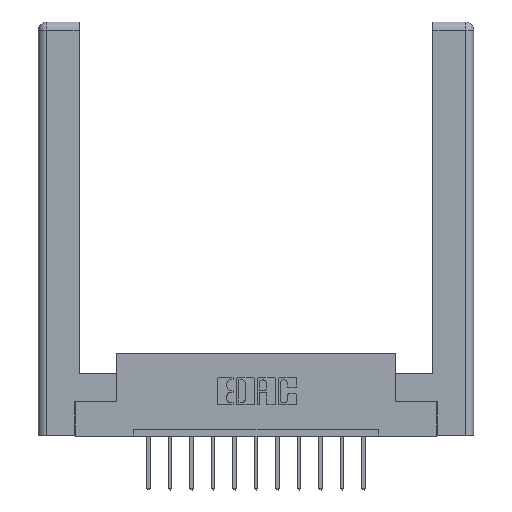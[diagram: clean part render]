
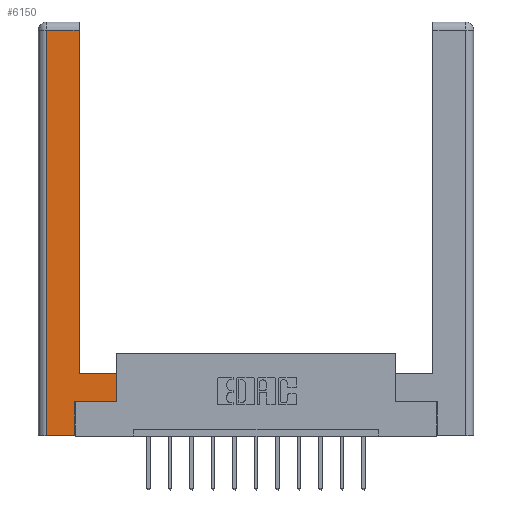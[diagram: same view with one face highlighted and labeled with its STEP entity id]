
A CAD part, top view. The second image highlights one B-rep face of the part: STEP entity #6150.
In plain terms, the highlighted planar face has unit normal (0, 0, 1).
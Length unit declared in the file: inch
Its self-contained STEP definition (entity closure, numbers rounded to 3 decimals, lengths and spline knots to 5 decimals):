
#1 = CARTESIAN_POINT ( 'NONE',  ( 0.295, 0.45, 0. ) ) ;
#195 = VERTEX_POINT ( 'NONE', #8451 ) ;
#566 = EDGE_CURVE ( 'NONE', #4747, #195, #12409, .T. ) ;
#671 = CARTESIAN_POINT ( 'NONE',  ( 0.565, 0.245, 0. ) ) ;
#918 = DIRECTION ( 'NONE',  ( -1., 0., 0. ) ) ;
#1179 = CARTESIAN_POINT ( 'NONE',  ( 0.265, 0.245, 0. ) ) ;
#1441 = EDGE_CURVE ( 'NONE', #195, #9207, #11475, .T. ) ;
#1463 = CARTESIAN_POINT ( 'NONE',  ( 0.0615, 0., 0. ) ) ;
#1494 = FACE_OUTER_BOUND ( 'NONE', #4042, .T. ) ;
#1576 = DIRECTION ( 'NONE',  ( 0., 1., 0. ) ) ;
#1592 = EDGE_CURVE ( 'NONE', #11965, #6570, #11661, .T. ) ;
#2027 = AXIS2_PLACEMENT_3D ( 'NONE', #5124, #5172, #2768 ) ;
#2190 = VECTOR ( 'NONE', #13616, 39.37008 ) ;
#2274 = EDGE_CURVE ( 'NONE', #11359, #4632, #4738, .T. ) ;
#2334 = VECTOR ( 'NONE', #12457, 39.37008 ) ;
#2402 = ORIENTED_EDGE ( 'NONE', *, *, #6427, .T. ) ;
#2768 = DIRECTION ( 'NONE',  ( -1., 0., 0. ) ) ;
#3490 = EDGE_CURVE ( 'NONE', #9207, #11965, #5975, .T. ) ;
#3733 = CARTESIAN_POINT ( 'NONE',  ( 0.295, 2.94, 0. ) ) ;
#4014 = ORIENTED_EDGE ( 'NONE', *, *, #566, .T. ) ;
#4042 = EDGE_LOOP ( 'NONE', ( #11072, #14363, #2402, #10550, #4014, #4528, #12501, #4617 ) ) ;
#4528 = ORIENTED_EDGE ( 'NONE', *, *, #1441, .T. ) ;
#4617 = ORIENTED_EDGE ( 'NONE', *, *, #1592, .T. ) ;
#4632 = VERTEX_POINT ( 'NONE', #6209 ) ;
#4738 = LINE ( 'NONE', #14704, #9374 ) ;
#4747 = VERTEX_POINT ( 'NONE', #6353 ) ;
#4816 = CARTESIAN_POINT ( 'NONE',  ( 0.295, 3., 0. ) ) ;
#4964 = LINE ( 'NONE', #6966, #10323 ) ;
#5046 = LINE ( 'NONE', #12704, #6117 ) ;
#5124 = CARTESIAN_POINT ( 'NONE',  ( 0., 0., 0. ) ) ;
#5172 = DIRECTION ( 'NONE',  ( 0., 0., -1. ) ) ;
#5835 = DIRECTION ( 'NONE',  ( 0., -1., 0. ) ) ;
#5836 = CARTESIAN_POINT ( 'NONE',  ( 0.565, 0.245, 0. ) ) ;
#5927 = PLANE ( 'NONE',  #2027 ) ;
#5975 = LINE ( 'NONE', #11966, #9903 ) ;
#6007 = CARTESIAN_POINT ( 'NONE',  ( 0.565, 0.45, 0. ) ) ;
#6117 = VECTOR ( 'NONE', #5835, 39.37008 ) ;
#6150 = ADVANCED_FACE ( 'NONE', ( #1494 ), #5927, .F. ) ;
#6209 = CARTESIAN_POINT ( 'NONE',  ( 0.0615, 2.94, 0. ) ) ;
#6353 = CARTESIAN_POINT ( 'NONE',  ( 0.265, 0., 0. ) ) ;
#6427 = EDGE_CURVE ( 'NONE', #4632, #9365, #5046, .T. ) ;
#6442 = VECTOR ( 'NONE', #7514, 39.37008 ) ;
#6570 = VERTEX_POINT ( 'NONE', #9885 ) ;
#6966 = CARTESIAN_POINT ( 'NONE',  ( 0.265, 0., 0. ) ) ;
#7514 = DIRECTION ( 'NONE',  ( 1., 0., 0. ) ) ;
#8451 = CARTESIAN_POINT ( 'NONE',  ( 0.265, 0.245, 0. ) ) ;
#9188 = VECTOR ( 'NONE', #9263, 39.37008 ) ;
#9207 = VERTEX_POINT ( 'NONE', #5836 ) ;
#9209 = EDGE_CURVE ( 'NONE', #6570, #11359, #12267, .T. ) ;
#9263 = DIRECTION ( 'NONE',  ( 0., 1., 0. ) ) ;
#9365 = VERTEX_POINT ( 'NONE', #1463 ) ;
#9374 = VECTOR ( 'NONE', #918, 39.37008 ) ;
#9885 = CARTESIAN_POINT ( 'NONE',  ( 0.295, 0.45, 0. ) ) ;
#9903 = VECTOR ( 'NONE', #1576, 39.37008 ) ;
#10323 = VECTOR ( 'NONE', #12722, 39.37008 ) ;
#10550 = ORIENTED_EDGE ( 'NONE', *, *, #14057, .T. ) ;
#11072 = ORIENTED_EDGE ( 'NONE', *, *, #9209, .T. ) ;
#11359 = VERTEX_POINT ( 'NONE', #3733 ) ;
#11475 = LINE ( 'NONE', #671, #6442 ) ;
#11661 = LINE ( 'NONE', #1, #2334 ) ;
#11965 = VERTEX_POINT ( 'NONE', #6007 ) ;
#11966 = CARTESIAN_POINT ( 'NONE',  ( 0.565, 0.45, 0. ) ) ;
#12267 = LINE ( 'NONE', #4816, #9188 ) ;
#12409 = LINE ( 'NONE', #1179, #2190 ) ;
#12457 = DIRECTION ( 'NONE',  ( -1., 0., 0. ) ) ;
#12501 = ORIENTED_EDGE ( 'NONE', *, *, #3490, .T. ) ;
#12704 = CARTESIAN_POINT ( 'NONE',  ( 0.0615, 0., 0. ) ) ;
#12722 = DIRECTION ( 'NONE',  ( 1., 0., 0. ) ) ;
#13616 = DIRECTION ( 'NONE',  ( 0., 1., 0. ) ) ;
#14057 = EDGE_CURVE ( 'NONE', #9365, #4747, #4964, .T. ) ;
#14363 = ORIENTED_EDGE ( 'NONE', *, *, #2274, .T. ) ;
#14704 = CARTESIAN_POINT ( 'NONE',  ( 0.0615, 2.94, 0. ) ) ;
